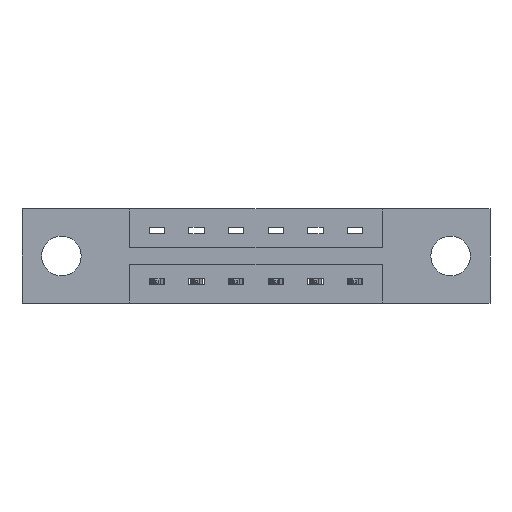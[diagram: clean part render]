
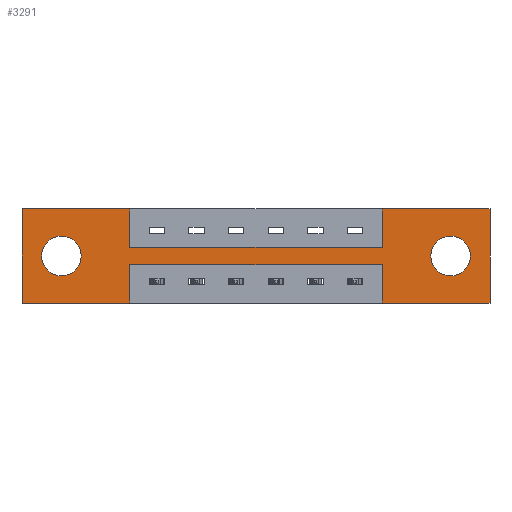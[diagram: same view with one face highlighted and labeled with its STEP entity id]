
A CAD part, front view. The second image highlights one B-rep face of the part: STEP entity #3291.
In plain terms, the highlighted planar face has unit normal (0, -1, 0).
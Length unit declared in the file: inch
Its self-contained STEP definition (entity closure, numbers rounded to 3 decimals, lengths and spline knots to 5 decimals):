
#111 = VECTOR ( 'NONE', #2427, 39.37008 ) ;
#195 = AXIS2_PLACEMENT_3D ( 'NONE', #4327, #7492, #7481 ) ;
#237 = AXIS2_PLACEMENT_3D ( 'NONE', #1948, #6718, #1636 ) ;
#254 = DIRECTION ( 'NONE',  ( -1., 0., 0. ) ) ;
#336 = CARTESIAN_POINT ( 'NONE',  ( 1.687, 0., -0.185 ) ) ;
#342 = EDGE_CURVE ( 'NONE', #6318, #8291, #7544, .T. ) ;
#350 = EDGE_LOOP ( 'NONE', ( #652, #7570, #6795, #7385, #2656, #788, #7769, #9145, #4338, #579, #3057, #8510 ) ) ;
#361 = DIRECTION ( 'NONE',  ( 0., 0., 1. ) ) ;
#449 = CARTESIAN_POINT ( 'NONE',  ( 0.155, 0., -0.263 ) ) ;
#532 = VERTEX_POINT ( 'NONE', #4244 ) ;
#579 = ORIENTED_EDGE ( 'NONE', *, *, #5492, .F. ) ;
#652 = ORIENTED_EDGE ( 'NONE', *, *, #2447, .F. ) ;
#744 = ORIENTED_EDGE ( 'NONE', *, *, #1946, .T. ) ;
#771 = CARTESIAN_POINT ( 'NONE',  ( 0.425, 0., 0. ) ) ;
#788 = ORIENTED_EDGE ( 'NONE', *, *, #2873, .F. ) ;
#824 = DIRECTION ( 'NONE',  ( -1., 0., 0. ) ) ;
#950 = CARTESIAN_POINT ( 'NONE',  ( 0., 0., -0.37 ) ) ;
#1011 = EDGE_CURVE ( 'NONE', #8291, #5702, #8284, .T. ) ;
#1070 = CARTESIAN_POINT ( 'NONE',  ( 1.842, 0., -0.37 ) ) ;
#1108 = CARTESIAN_POINT ( 'NONE',  ( 0., 0., 0. ) ) ;
#1172 = CARTESIAN_POINT ( 'NONE',  ( 0.425, 0., 0. ) ) ;
#1254 = CARTESIAN_POINT ( 'NONE',  ( 1.687, 0., -0.185 ) ) ;
#1357 = FACE_OUTER_BOUND ( 'NONE', #350, .T. ) ;
#1378 = LINE ( 'NONE', #7914, #3615 ) ;
#1413 = VERTEX_POINT ( 'NONE', #4555 ) ;
#1415 = EDGE_CURVE ( 'NONE', #6408, #6155, #4185, .T. ) ;
#1443 = DIRECTION ( 'NONE',  ( 0., 0., 1. ) ) ;
#1473 = CARTESIAN_POINT ( 'NONE',  ( 1.417, 0., 0. ) ) ;
#1486 = DIRECTION ( 'NONE',  ( 1., 0., 0. ) ) ;
#1491 = CARTESIAN_POINT ( 'NONE',  ( 0.425, 0., -0.37 ) ) ;
#1519 = DIRECTION ( 'NONE',  ( 0., 0., -1. ) ) ;
#1569 = LINE ( 'NONE', #771, #7024 ) ;
#1636 = DIRECTION ( 'NONE',  ( 0., 0., 1. ) ) ;
#1862 = LINE ( 'NONE', #8384, #4136 ) ;
#1901 = VECTOR ( 'NONE', #254, 39.37008 ) ;
#1919 = PLANE ( 'NONE',  #195 ) ;
#1946 = EDGE_CURVE ( 'NONE', #2805, #8067, #7185, .T. ) ;
#1948 = CARTESIAN_POINT ( 'NONE',  ( 0.155, 0., -0.185 ) ) ;
#2014 = CARTESIAN_POINT ( 'NONE',  ( 0.425, 0., -0.22 ) ) ;
#2030 = DIRECTION ( 'NONE',  ( 0., 0., -1. ) ) ;
#2081 = EDGE_CURVE ( 'NONE', #6309, #4648, #8902, .T. ) ;
#2309 = VERTEX_POINT ( 'NONE', #2014 ) ;
#2427 = DIRECTION ( 'NONE',  ( 0., 0., -1. ) ) ;
#2428 = ORIENTED_EDGE ( 'NONE', *, *, #6192, .T. ) ;
#2442 = CARTESIAN_POINT ( 'NONE',  ( 1.417, 0., -0.37 ) ) ;
#2447 = EDGE_CURVE ( 'NONE', #2309, #6408, #6381, .T. ) ;
#2570 = DIRECTION ( 'NONE',  ( 0., 0., -1. ) ) ;
#2622 = EDGE_CURVE ( 'NONE', #2759, #2309, #6981, .T. ) ;
#2656 = ORIENTED_EDGE ( 'NONE', *, *, #342, .F. ) ;
#2759 = VERTEX_POINT ( 'NONE', #2867 ) ;
#2805 = VERTEX_POINT ( 'NONE', #4766 ) ;
#2867 = CARTESIAN_POINT ( 'NONE',  ( 1.417, 0., -0.22 ) ) ;
#2873 = EDGE_CURVE ( 'NONE', #532, #6318, #1862, .T. ) ;
#2903 = EDGE_CURVE ( 'NONE', #5702, #2759, #1378, .T. ) ;
#2904 = EDGE_LOOP ( 'NONE', ( #5016, #8612 ) ) ;
#3019 = EDGE_LOOP ( 'NONE', ( #744, #2428 ) ) ;
#3057 = ORIENTED_EDGE ( 'NONE', *, *, #6996, .F. ) ;
#3291 = ADVANCED_FACE ( 'NONE', ( #7241, #8666, #1357 ), #1919, .T. ) ;
#3400 = VERTEX_POINT ( 'NONE', #7253 ) ;
#3615 = VECTOR ( 'NONE', #361, 39.37008 ) ;
#3943 = EDGE_CURVE ( 'NONE', #3400, #532, #7214, .T. ) ;
#3960 = CARTESIAN_POINT ( 'NONE',  ( 0.155, 0., -0.185 ) ) ;
#4077 = LINE ( 'NONE', #6720, #5487 ) ;
#4136 = VECTOR ( 'NONE', #8378, 39.37008 ) ;
#4185 = LINE ( 'NONE', #8596, #1901 ) ;
#4244 = CARTESIAN_POINT ( 'NONE',  ( 1.417, 0., 0. ) ) ;
#4327 = CARTESIAN_POINT ( 'NONE',  ( 0., 0., -0.37 ) ) ;
#4338 = ORIENTED_EDGE ( 'NONE', *, *, #5218, .F. ) ;
#4555 = CARTESIAN_POINT ( 'NONE',  ( 0.425, 0., -0.15 ) ) ;
#4648 = VERTEX_POINT ( 'NONE', #449 ) ;
#4712 = DIRECTION ( 'NONE',  ( 0., 0., 1. ) ) ;
#4766 = CARTESIAN_POINT ( 'NONE',  ( 1.687, 0., -0.107 ) ) ;
#4817 = CIRCLE ( 'NONE', #6470, 0.078 ) ;
#4965 = CARTESIAN_POINT ( 'NONE',  ( 0.425, 0., -0.22 ) ) ;
#5016 = ORIENTED_EDGE ( 'NONE', *, *, #2081, .T. ) ;
#5207 = EDGE_CURVE ( 'NONE', #1413, #3400, #4077, .T. ) ;
#5218 = EDGE_CURVE ( 'NONE', #8414, #1413, #1569, .T. ) ;
#5245 = VECTOR ( 'NONE', #5481, 39.37008 ) ;
#5481 = DIRECTION ( 'NONE',  ( -1., 0., 0. ) ) ;
#5487 = VECTOR ( 'NONE', #1486, 39.37008 ) ;
#5492 = EDGE_CURVE ( 'NONE', #5861, #8414, #8229, .T. ) ;
#5660 = CARTESIAN_POINT ( 'NONE',  ( 0., 0., 0. ) ) ;
#5702 = VERTEX_POINT ( 'NONE', #2442 ) ;
#5861 = VERTEX_POINT ( 'NONE', #5660 ) ;
#5982 = CARTESIAN_POINT ( 'NONE',  ( 1.842, 0., 0. ) ) ;
#6155 = VERTEX_POINT ( 'NONE', #8931 ) ;
#6192 = EDGE_CURVE ( 'NONE', #8067, #2805, #4817, .T. ) ;
#6309 = VERTEX_POINT ( 'NONE', #9075 ) ;
#6318 = VERTEX_POINT ( 'NONE', #5982 ) ;
#6344 = EDGE_CURVE ( 'NONE', #4648, #6309, #6874, .T. ) ;
#6381 = LINE ( 'NONE', #8005, #111 ) ;
#6408 = VERTEX_POINT ( 'NONE', #1491 ) ;
#6470 = AXIS2_PLACEMENT_3D ( 'NONE', #1254, #6534, #2030 ) ;
#6534 = DIRECTION ( 'NONE',  ( 0., 1., 0. ) ) ;
#6644 = VECTOR ( 'NONE', #824, 39.37008 ) ;
#6660 = VECTOR ( 'NONE', #7685, 39.37008 ) ;
#6718 = DIRECTION ( 'NONE',  ( 0., 1., 0. ) ) ;
#6720 = CARTESIAN_POINT ( 'NONE',  ( 0.425, 0., -0.15 ) ) ;
#6763 = CARTESIAN_POINT ( 'NONE',  ( 0., 0., 0. ) ) ;
#6795 = ORIENTED_EDGE ( 'NONE', *, *, #2903, .F. ) ;
#6832 = CARTESIAN_POINT ( 'NONE',  ( 1.687, 0., -0.263 ) ) ;
#6874 = CIRCLE ( 'NONE', #7740, 0.078 ) ;
#6981 = LINE ( 'NONE', #4965, #5245 ) ;
#6996 = EDGE_CURVE ( 'NONE', #6155, #5861, #8306, .T. ) ;
#7024 = VECTOR ( 'NONE', #1519, 39.37008 ) ;
#7073 = DIRECTION ( 'NONE',  ( 0., 0., -1. ) ) ;
#7154 = VECTOR ( 'NONE', #7073, 39.37008 ) ;
#7185 = CIRCLE ( 'NONE', #7759, 0.078 ) ;
#7214 = LINE ( 'NONE', #1473, #8837 ) ;
#7241 = FACE_BOUND ( 'NONE', #3019, .T. ) ;
#7253 = CARTESIAN_POINT ( 'NONE',  ( 1.417, 0., -0.15 ) ) ;
#7256 = DIRECTION ( 'NONE',  ( 0., 1., 0. ) ) ;
#7385 = ORIENTED_EDGE ( 'NONE', *, *, #1011, .F. ) ;
#7392 = DIRECTION ( 'NONE',  ( 1., 0., 0. ) ) ;
#7481 = DIRECTION ( 'NONE',  ( 0., 0., -1. ) ) ;
#7492 = DIRECTION ( 'NONE',  ( 0., -1., 0. ) ) ;
#7544 = LINE ( 'NONE', #8408, #7154 ) ;
#7570 = ORIENTED_EDGE ( 'NONE', *, *, #2622, .F. ) ;
#7685 = DIRECTION ( 'NONE',  ( 0., 0., 1. ) ) ;
#7740 = AXIS2_PLACEMENT_3D ( 'NONE', #3960, #8528, #4712 ) ;
#7759 = AXIS2_PLACEMENT_3D ( 'NONE', #336, #7256, #2570 ) ;
#7769 = ORIENTED_EDGE ( 'NONE', *, *, #3943, .F. ) ;
#7914 = CARTESIAN_POINT ( 'NONE',  ( 1.417, 0., -0.37 ) ) ;
#8005 = CARTESIAN_POINT ( 'NONE',  ( 0.425, 0., -0.37 ) ) ;
#8034 = VECTOR ( 'NONE', #7392, 39.37008 ) ;
#8067 = VERTEX_POINT ( 'NONE', #6832 ) ;
#8229 = LINE ( 'NONE', #6763, #8034 ) ;
#8284 = LINE ( 'NONE', #950, #6644 ) ;
#8291 = VERTEX_POINT ( 'NONE', #1070 ) ;
#8306 = LINE ( 'NONE', #1108, #6660 ) ;
#8378 = DIRECTION ( 'NONE',  ( 1., 0., 0. ) ) ;
#8384 = CARTESIAN_POINT ( 'NONE',  ( 0., 0., 0. ) ) ;
#8408 = CARTESIAN_POINT ( 'NONE',  ( 1.842, 0., 0. ) ) ;
#8414 = VERTEX_POINT ( 'NONE', #1172 ) ;
#8510 = ORIENTED_EDGE ( 'NONE', *, *, #1415, .F. ) ;
#8528 = DIRECTION ( 'NONE',  ( 0., 1., 0. ) ) ;
#8596 = CARTESIAN_POINT ( 'NONE',  ( 0., 0., -0.37 ) ) ;
#8612 = ORIENTED_EDGE ( 'NONE', *, *, #6344, .T. ) ;
#8666 = FACE_BOUND ( 'NONE', #2904, .T. ) ;
#8837 = VECTOR ( 'NONE', #1443, 39.37008 ) ;
#8902 = CIRCLE ( 'NONE', #237, 0.078 ) ;
#8931 = CARTESIAN_POINT ( 'NONE',  ( 0., 0., -0.37 ) ) ;
#9075 = CARTESIAN_POINT ( 'NONE',  ( 0.155, 0., -0.107 ) ) ;
#9145 = ORIENTED_EDGE ( 'NONE', *, *, #5207, .F. ) ;
